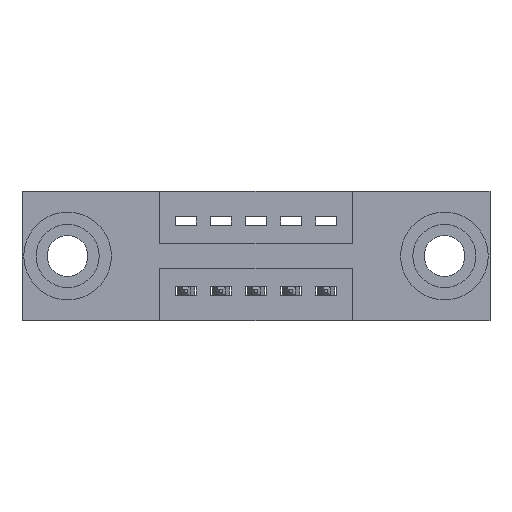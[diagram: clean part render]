
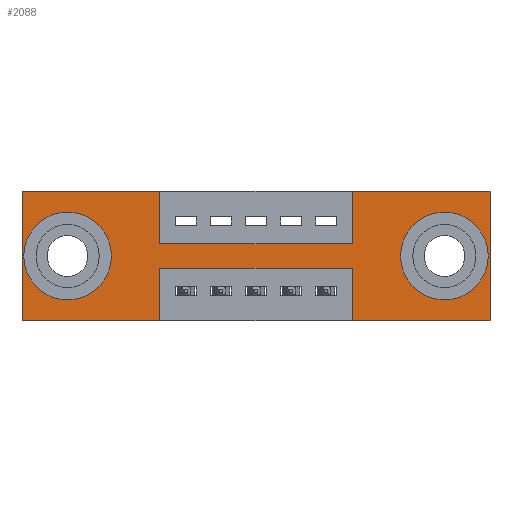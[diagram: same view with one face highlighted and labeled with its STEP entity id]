
A CAD part, front view. The second image highlights one B-rep face of the part: STEP entity #2088.
In plain terms, the highlighted planar face has unit normal (0, -1, 0).
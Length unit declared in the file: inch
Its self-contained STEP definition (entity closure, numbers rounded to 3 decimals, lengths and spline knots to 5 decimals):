
#97 = DIRECTION ( 'NONE',  ( 0., 0., -1. ) ) ;
#108 = DIRECTION ( 'NONE',  ( 0., 0., -1. ) ) ;
#171 = EDGE_CURVE ( 'NONE', #3817, #8232, #4695, .T. ) ;
#182 = ORIENTED_EDGE ( 'NONE', *, *, #171, .F. ) ;
#194 = LINE ( 'NONE', #977, #9287 ) ;
#198 = CARTESIAN_POINT ( 'NONE',  ( 0., 0., 0. ) ) ;
#248 = CARTESIAN_POINT ( 'NONE',  ( 0.9425, 0., -0.15 ) ) ;
#291 = DIRECTION ( 'NONE',  ( 0., 0., -1. ) ) ;
#359 = FACE_BOUND ( 'NONE', #2519, .T. ) ;
#439 = DIRECTION ( 'NONE',  ( -1., 0., 0. ) ) ;
#607 = CARTESIAN_POINT ( 'NONE',  ( 0.13, 0., -0.107 ) ) ;
#682 = LINE ( 'NONE', #4759, #8976 ) ;
#808 = EDGE_CURVE ( 'NONE', #4100, #7097, #6656, .T. ) ;
#888 = LINE ( 'NONE', #1909, #5427 ) ;
#960 = CARTESIAN_POINT ( 'NONE',  ( 1.335, 0., 0. ) ) ;
#977 = CARTESIAN_POINT ( 'NONE',  ( 0.3925, 0., -0.15 ) ) ;
#1035 = CIRCLE ( 'NONE', #4435, 0.078 ) ;
#1103 = ORIENTED_EDGE ( 'NONE', *, *, #9292, .F. ) ;
#1142 = VERTEX_POINT ( 'NONE', #4621 ) ;
#1154 = CARTESIAN_POINT ( 'NONE',  ( 0.3925, 0., -0.37 ) ) ;
#1193 = VERTEX_POINT ( 'NONE', #3278 ) ;
#1237 = DIRECTION ( 'NONE',  ( 0., 0., 1. ) ) ;
#1313 = ORIENTED_EDGE ( 'NONE', *, *, #2876, .T. ) ;
#1318 = DIRECTION ( 'NONE',  ( 0., 0., 1. ) ) ;
#1360 = ORIENTED_EDGE ( 'NONE', *, *, #4540, .F. ) ;
#1469 = VECTOR ( 'NONE', #8401, 39.37008 ) ;
#1542 = DIRECTION ( 'NONE',  ( 0., 1., 0. ) ) ;
#1606 = CIRCLE ( 'NONE', #3135, 0.078 ) ;
#1823 = VERTEX_POINT ( 'NONE', #7320 ) ;
#1896 = CARTESIAN_POINT ( 'NONE',  ( 0.9425, 0., -0.22 ) ) ;
#1908 = PLANE ( 'NONE',  #3520 ) ;
#1909 = CARTESIAN_POINT ( 'NONE',  ( 0., 0., -0.37 ) ) ;
#2088 = ADVANCED_FACE ( 'NONE', ( #9012, #359, #5704 ), #1908, .T. ) ;
#2106 = CARTESIAN_POINT ( 'NONE',  ( 0., 0., 0. ) ) ;
#2227 = DIRECTION ( 'NONE',  ( -1., 0., 0. ) ) ;
#2519 = EDGE_LOOP ( 'NONE', ( #5795, #8021 ) ) ;
#2611 = LINE ( 'NONE', #9127, #1469 ) ;
#2638 = CARTESIAN_POINT ( 'NONE',  ( 0.9425, 0., 0. ) ) ;
#2876 = EDGE_CURVE ( 'NONE', #3907, #7597, #7651, .T. ) ;
#3080 = EDGE_CURVE ( 'NONE', #8807, #1823, #7416, .T. ) ;
#3132 = EDGE_CURVE ( 'NONE', #7597, #3907, #1606, .T. ) ;
#3135 = AXIS2_PLACEMENT_3D ( 'NONE', #4033, #6897, #291 ) ;
#3151 = ORIENTED_EDGE ( 'NONE', *, *, #3677, .F. ) ;
#3154 = LINE ( 'NONE', #8092, #6590 ) ;
#3278 = CARTESIAN_POINT ( 'NONE',  ( 0.3925, 0., -0.15 ) ) ;
#3284 = VERTEX_POINT ( 'NONE', #2638 ) ;
#3430 = ORIENTED_EDGE ( 'NONE', *, *, #3651, .F. ) ;
#3456 = VERTEX_POINT ( 'NONE', #607 ) ;
#3460 = CARTESIAN_POINT ( 'NONE',  ( 1.335, 0., -0.37 ) ) ;
#3520 = AXIS2_PLACEMENT_3D ( 'NONE', #5519, #5550, #7700 ) ;
#3651 = EDGE_CURVE ( 'NONE', #8232, #1193, #2611, .T. ) ;
#3677 = EDGE_CURVE ( 'NONE', #4576, #8807, #682, .T. ) ;
#3817 = VERTEX_POINT ( 'NONE', #7080 ) ;
#3836 = DIRECTION ( 'NONE',  ( 1., 0., 0. ) ) ;
#3883 = ORIENTED_EDGE ( 'NONE', *, *, #5043, .F. ) ;
#3907 = VERTEX_POINT ( 'NONE', #7858 ) ;
#3955 = LINE ( 'NONE', #5834, #7509 ) ;
#3995 = DIRECTION ( 'NONE',  ( 0., 0., -1. ) ) ;
#4007 = ORIENTED_EDGE ( 'NONE', *, *, #3080, .F. ) ;
#4022 = DIRECTION ( 'NONE',  ( 0., 0., 1. ) ) ;
#4033 = CARTESIAN_POINT ( 'NONE',  ( 1.205, 0., -0.185 ) ) ;
#4093 = DIRECTION ( 'NONE',  ( 0., 1., 0. ) ) ;
#4100 = VERTEX_POINT ( 'NONE', #5902 ) ;
#4237 = EDGE_CURVE ( 'NONE', #8051, #3284, #3955, .T. ) ;
#4290 = VECTOR ( 'NONE', #2227, 39.37008 ) ;
#4362 = ORIENTED_EDGE ( 'NONE', *, *, #5111, .F. ) ;
#4435 = AXIS2_PLACEMENT_3D ( 'NONE', #4928, #1542, #1318 ) ;
#4540 = EDGE_CURVE ( 'NONE', #7016, #8462, #888, .T. ) ;
#4576 = VERTEX_POINT ( 'NONE', #5483 ) ;
#4599 = AXIS2_PLACEMENT_3D ( 'NONE', #8553, #4093, #1237 ) ;
#4621 = CARTESIAN_POINT ( 'NONE',  ( 0.13, 0., -0.263 ) ) ;
#4695 = LINE ( 'NONE', #198, #6197 ) ;
#4759 = CARTESIAN_POINT ( 'NONE',  ( 0.9425, 0., -0.37 ) ) ;
#4770 = EDGE_CURVE ( 'NONE', #3456, #1142, #9302, .T. ) ;
#4781 = CARTESIAN_POINT ( 'NONE',  ( 1.205, 0., -0.107 ) ) ;
#4928 = CARTESIAN_POINT ( 'NONE',  ( 0.13, 0., -0.185 ) ) ;
#4935 = VECTOR ( 'NONE', #3995, 39.37008 ) ;
#5043 = EDGE_CURVE ( 'NONE', #7097, #4576, #6237, .T. ) ;
#5065 = ORIENTED_EDGE ( 'NONE', *, *, #808, .F. ) ;
#5111 = EDGE_CURVE ( 'NONE', #1193, #8051, #194, .T. ) ;
#5180 = DIRECTION ( 'NONE',  ( 0., 1., 0. ) ) ;
#5302 = DIRECTION ( 'NONE',  ( 1., 0., 0. ) ) ;
#5427 = VECTOR ( 'NONE', #439, 39.37008 ) ;
#5442 = ORIENTED_EDGE ( 'NONE', *, *, #4237, .F. ) ;
#5483 = CARTESIAN_POINT ( 'NONE',  ( 0.9425, 0., -0.37 ) ) ;
#5519 = CARTESIAN_POINT ( 'NONE',  ( 0., 0., -0.37 ) ) ;
#5550 = DIRECTION ( 'NONE',  ( 0., -1., 0. ) ) ;
#5698 = LINE ( 'NONE', #2106, #8327 ) ;
#5704 = FACE_OUTER_BOUND ( 'NONE', #6382, .T. ) ;
#5795 = ORIENTED_EDGE ( 'NONE', *, *, #4770, .T. ) ;
#5819 = CARTESIAN_POINT ( 'NONE',  ( 1.205, 0., -0.185 ) ) ;
#5828 = ORIENTED_EDGE ( 'NONE', *, *, #3132, .T. ) ;
#5834 = CARTESIAN_POINT ( 'NONE',  ( 0.9425, 0., 0. ) ) ;
#5902 = CARTESIAN_POINT ( 'NONE',  ( 1.335, 0., 0. ) ) ;
#5998 = CARTESIAN_POINT ( 'NONE',  ( 0., 0., -0.37 ) ) ;
#6067 = DIRECTION ( 'NONE',  ( 1., 0., 0. ) ) ;
#6079 = EDGE_CURVE ( 'NONE', #8462, #3817, #5698, .T. ) ;
#6197 = VECTOR ( 'NONE', #5302, 39.37008 ) ;
#6237 = LINE ( 'NONE', #5998, #4290 ) ;
#6359 = LINE ( 'NONE', #7462, #7835 ) ;
#6382 = EDGE_LOOP ( 'NONE', ( #7245, #4007, #3151, #3883, #5065, #1103, #5442, #4362, #3430, #182, #9061, #1360 ) ) ;
#6528 = EDGE_CURVE ( 'NONE', #1142, #3456, #1035, .T. ) ;
#6590 = VECTOR ( 'NONE', #97, 39.37008 ) ;
#6656 = LINE ( 'NONE', #960, #4935 ) ;
#6705 = EDGE_LOOP ( 'NONE', ( #5828, #1313 ) ) ;
#6783 = CARTESIAN_POINT ( 'NONE',  ( 0.3925, 0., -0.22 ) ) ;
#6897 = DIRECTION ( 'NONE',  ( 0., 1., 0. ) ) ;
#7016 = VERTEX_POINT ( 'NONE', #1154 ) ;
#7058 = DIRECTION ( 'NONE',  ( 0., 0., 1. ) ) ;
#7080 = CARTESIAN_POINT ( 'NONE',  ( 0., 0., 0. ) ) ;
#7092 = DIRECTION ( 'NONE',  ( 0., 0., 1. ) ) ;
#7097 = VERTEX_POINT ( 'NONE', #3460 ) ;
#7245 = ORIENTED_EDGE ( 'NONE', *, *, #8005, .F. ) ;
#7320 = CARTESIAN_POINT ( 'NONE',  ( 0.3925, 0., -0.22 ) ) ;
#7416 = LINE ( 'NONE', #6783, #8664 ) ;
#7462 = CARTESIAN_POINT ( 'NONE',  ( 0., 0., 0. ) ) ;
#7463 = DIRECTION ( 'NONE',  ( -1., 0., 0. ) ) ;
#7509 = VECTOR ( 'NONE', #7058, 39.37008 ) ;
#7597 = VERTEX_POINT ( 'NONE', #4781 ) ;
#7651 = CIRCLE ( 'NONE', #8152, 0.078 ) ;
#7700 = DIRECTION ( 'NONE',  ( 0., 0., -1. ) ) ;
#7835 = VECTOR ( 'NONE', #3836, 39.37008 ) ;
#7858 = CARTESIAN_POINT ( 'NONE',  ( 1.205, 0., -0.263 ) ) ;
#8005 = EDGE_CURVE ( 'NONE', #1823, #7016, #3154, .T. ) ;
#8021 = ORIENTED_EDGE ( 'NONE', *, *, #6528, .T. ) ;
#8051 = VERTEX_POINT ( 'NONE', #248 ) ;
#8092 = CARTESIAN_POINT ( 'NONE',  ( 0.3925, 0., -0.37 ) ) ;
#8152 = AXIS2_PLACEMENT_3D ( 'NONE', #5819, #5180, #108 ) ;
#8232 = VERTEX_POINT ( 'NONE', #8398 ) ;
#8327 = VECTOR ( 'NONE', #7092, 39.37008 ) ;
#8398 = CARTESIAN_POINT ( 'NONE',  ( 0.3925, 0., 0. ) ) ;
#8401 = DIRECTION ( 'NONE',  ( 0., 0., -1. ) ) ;
#8462 = VERTEX_POINT ( 'NONE', #9408 ) ;
#8553 = CARTESIAN_POINT ( 'NONE',  ( 0.13, 0., -0.185 ) ) ;
#8664 = VECTOR ( 'NONE', #7463, 39.37008 ) ;
#8807 = VERTEX_POINT ( 'NONE', #1896 ) ;
#8976 = VECTOR ( 'NONE', #4022, 39.37008 ) ;
#9012 = FACE_BOUND ( 'NONE', #6705, .T. ) ;
#9061 = ORIENTED_EDGE ( 'NONE', *, *, #6079, .F. ) ;
#9127 = CARTESIAN_POINT ( 'NONE',  ( 0.3925, 0., 0. ) ) ;
#9287 = VECTOR ( 'NONE', #6067, 39.37008 ) ;
#9292 = EDGE_CURVE ( 'NONE', #3284, #4100, #6359, .T. ) ;
#9302 = CIRCLE ( 'NONE', #4599, 0.078 ) ;
#9408 = CARTESIAN_POINT ( 'NONE',  ( 0., 0., -0.37 ) ) ;
